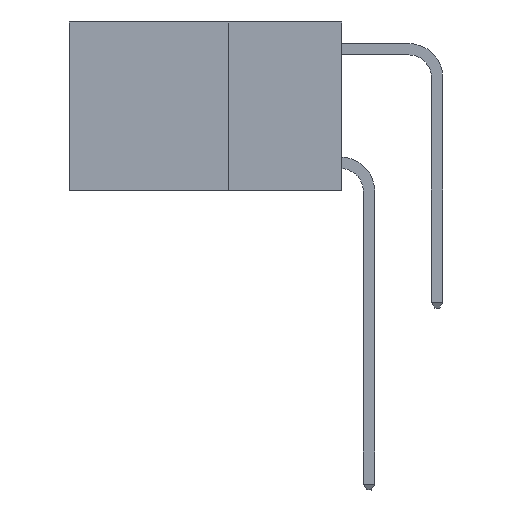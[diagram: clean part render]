
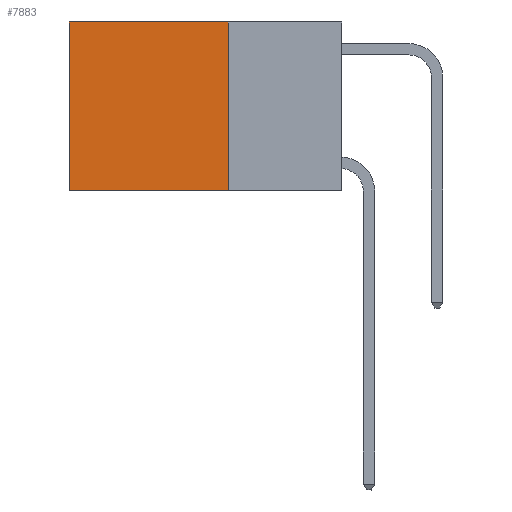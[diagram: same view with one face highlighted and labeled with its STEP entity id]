
A CAD part, left-side view. The second image highlights one B-rep face of the part: STEP entity #7883.
In plain terms, the highlighted planar face has unit normal (-1, 0, 0).
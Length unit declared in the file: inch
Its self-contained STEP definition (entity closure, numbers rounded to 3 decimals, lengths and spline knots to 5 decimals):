
#760 = CARTESIAN_POINT ( 'NONE',  ( 0.2625, 0.6, 0. ) ) ;
#1065 = DIRECTION ( 'NONE',  ( 0., 0., -1. ) ) ;
#1849 = CARTESIAN_POINT ( 'NONE',  ( 0.2625, 0.25, -0.37 ) ) ;
#2808 = EDGE_CURVE ( 'NONE', #5141, #10543, #11919, .T. ) ;
#2828 = DIRECTION ( 'NONE',  ( 0., 1., 0. ) ) ;
#2971 = PLANE ( 'NONE',  #7514 ) ;
#3097 = DIRECTION ( 'NONE',  ( 0., 0., -1. ) ) ;
#3154 = EDGE_CURVE ( 'NONE', #10543, #5125, #7493, .T. ) ;
#3484 = DIRECTION ( 'NONE',  ( 0., 1., 0. ) ) ;
#3579 = ORIENTED_EDGE ( 'NONE', *, *, #3154, .F. ) ;
#4941 = VECTOR ( 'NONE', #3097, 39.37008 ) ;
#5125 = VERTEX_POINT ( 'NONE', #9985 ) ;
#5141 = VERTEX_POINT ( 'NONE', #8840 ) ;
#5156 = ORIENTED_EDGE ( 'NONE', *, *, #12507, .T. ) ;
#5175 = CARTESIAN_POINT ( 'NONE',  ( 0.2625, 0.25, 0. ) ) ;
#5601 = VECTOR ( 'NONE', #2828, 39.37008 ) ;
#5795 = VERTEX_POINT ( 'NONE', #11153 ) ;
#5990 = LINE ( 'NONE', #760, #4941 ) ;
#6823 = CARTESIAN_POINT ( 'NONE',  ( 0.2625, 0.25, 0. ) ) ;
#7493 = LINE ( 'NONE', #1849, #5601 ) ;
#7514 = AXIS2_PLACEMENT_3D ( 'NONE', #5175, #9328, #9375 ) ;
#7661 = CARTESIAN_POINT ( 'NONE',  ( 0.2625, 0.25, 0. ) ) ;
#7883 = ADVANCED_FACE ( 'NONE', ( #8163 ), #2971, .F. ) ;
#8093 = LINE ( 'NONE', #6823, #13711 ) ;
#8163 = FACE_OUTER_BOUND ( 'NONE', #10257, .T. ) ;
#8686 = VECTOR ( 'NONE', #1065, 39.37008 ) ;
#8840 = CARTESIAN_POINT ( 'NONE',  ( 0.2625, 0.25, 0. ) ) ;
#9328 = DIRECTION ( 'NONE',  ( 1., 0., 0. ) ) ;
#9375 = DIRECTION ( 'NONE',  ( 0., 0., -1. ) ) ;
#9985 = CARTESIAN_POINT ( 'NONE',  ( 0.2625, 0.6, -0.37 ) ) ;
#10257 = EDGE_LOOP ( 'NONE', ( #5156, #3579, #12514, #14121 ) ) ;
#10543 = VERTEX_POINT ( 'NONE', #13161 ) ;
#10651 = EDGE_CURVE ( 'NONE', #5141, #5795, #8093, .T. ) ;
#11153 = CARTESIAN_POINT ( 'NONE',  ( 0.2625, 0.6, 0. ) ) ;
#11919 = LINE ( 'NONE', #7661, #8686 ) ;
#12507 = EDGE_CURVE ( 'NONE', #5795, #5125, #5990, .T. ) ;
#12514 = ORIENTED_EDGE ( 'NONE', *, *, #2808, .F. ) ;
#13161 = CARTESIAN_POINT ( 'NONE',  ( 0.2625, 0.25, -0.37 ) ) ;
#13711 = VECTOR ( 'NONE', #3484, 39.37008 ) ;
#14121 = ORIENTED_EDGE ( 'NONE', *, *, #10651, .T. ) ;
